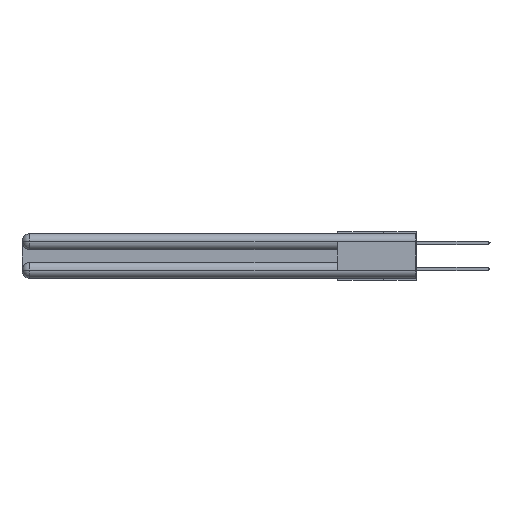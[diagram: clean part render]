
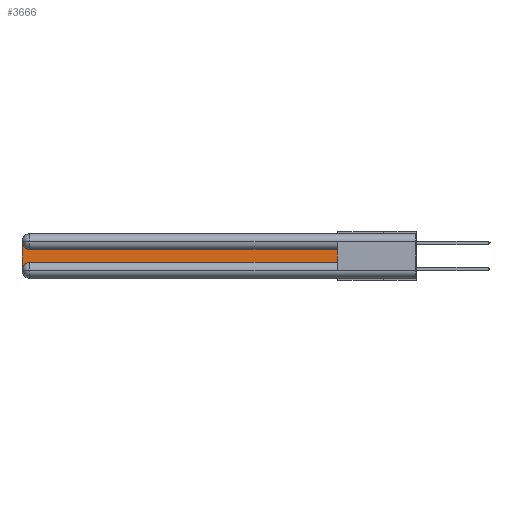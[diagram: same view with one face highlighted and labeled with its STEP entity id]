
A CAD part, left-side view. The second image highlights one B-rep face of the part: STEP entity #3666.
In plain terms, the highlighted planar face has unit normal (-1, 0, 0).
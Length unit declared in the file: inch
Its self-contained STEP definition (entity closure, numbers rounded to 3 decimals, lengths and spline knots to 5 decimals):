
#105 = CARTESIAN_POINT ( 'NONE',  ( 0.075, 2.94, -0.2775 ) ) ;
#425 = CIRCLE ( 'NONE', #22942, 0.06 ) ;
#796 = EDGE_CURVE ( 'NONE', #21981, #18552, #19063, .T. ) ;
#1457 = CARTESIAN_POINT ( 'NONE',  ( 0.075, 0.6, -0.2175 ) ) ;
#1483 = ORIENTED_EDGE ( 'NONE', *, *, #12545, .T. ) ;
#2326 = PLANE ( 'NONE',  #20164 ) ;
#3666 = ADVANCED_FACE ( 'NONE', ( #7728 ), #2326, .F. ) ;
#4022 = LINE ( 'NONE', #29807, #31252 ) ;
#4685 = DIRECTION ( 'NONE',  ( 0., 0., 1. ) ) ;
#5792 = DIRECTION ( 'NONE',  ( 1., 0., 0. ) ) ;
#7728 = FACE_OUTER_BOUND ( 'NONE', #14216, .T. ) ;
#8136 = EDGE_CURVE ( 'NONE', #31898, #27687, #425, .T. ) ;
#9173 = ORIENTED_EDGE ( 'NONE', *, *, #28149, .T. ) ;
#10000 = ORIENTED_EDGE ( 'NONE', *, *, #17375, .T. ) ;
#10413 = DIRECTION ( 'NONE',  ( 0., 0., -1. ) ) ;
#10922 = CARTESIAN_POINT ( 'NONE',  ( 0.075, 2.94, -0.2175 ) ) ;
#12545 = EDGE_CURVE ( 'NONE', #21343, #21981, #31211, .T. ) ;
#14216 = EDGE_LOOP ( 'NONE', ( #10000, #31484, #20580, #1483, #27017, #9173 ) ) ;
#15577 = DIRECTION ( 'NONE',  ( 1., 0., 0. ) ) ;
#16158 = CARTESIAN_POINT ( 'NONE',  ( 0.075, 0.6, -0.1225 ) ) ;
#17375 = EDGE_CURVE ( 'NONE', #26164, #31898, #23611, .T. ) ;
#18552 = VERTEX_POINT ( 'NONE', #1457 ) ;
#18980 = DIRECTION ( 'NONE',  ( 0., -1., 0. ) ) ;
#19063 = LINE ( 'NONE', #24415, #30120 ) ;
#19145 = DIRECTION ( 'NONE',  ( 0., 0., -1. ) ) ;
#19753 = CARTESIAN_POINT ( 'NONE',  ( 0.075, 3., -0.2775 ) ) ;
#19995 = CARTESIAN_POINT ( 'NONE',  ( 0.075, 3., -0.2175 ) ) ;
#20120 = DIRECTION ( 'NONE',  ( 0., 0., -1. ) ) ;
#20164 = AXIS2_PLACEMENT_3D ( 'NONE', #32639, #32169, #10413 ) ;
#20580 = ORIENTED_EDGE ( 'NONE', *, *, #24477, .T. ) ;
#21343 = VERTEX_POINT ( 'NONE', #19753 ) ;
#21544 = CARTESIAN_POINT ( 'NONE',  ( 0.075, 0.6, -0.1225 ) ) ;
#21981 = VERTEX_POINT ( 'NONE', #10922 ) ;
#22942 = AXIS2_PLACEMENT_3D ( 'NONE', #23781, #15577, #34905 ) ;
#23611 = LINE ( 'NONE', #16158, #25318 ) ;
#23781 = CARTESIAN_POINT ( 'NONE',  ( 0.075, 2.94, -0.0625 ) ) ;
#24415 = CARTESIAN_POINT ( 'NONE',  ( 0.075, 0.6, -0.2175 ) ) ;
#24477 = EDGE_CURVE ( 'NONE', #27687, #21343, #34116, .T. ) ;
#25318 = VECTOR ( 'NONE', #34889, 39.37008 ) ;
#25767 = AXIS2_PLACEMENT_3D ( 'NONE', #105, #5792, #19145 ) ;
#26164 = VERTEX_POINT ( 'NONE', #21544 ) ;
#27017 = ORIENTED_EDGE ( 'NONE', *, *, #796, .T. ) ;
#27687 = VERTEX_POINT ( 'NONE', #28642 ) ;
#28149 = EDGE_CURVE ( 'NONE', #18552, #26164, #4022, .T. ) ;
#28642 = CARTESIAN_POINT ( 'NONE',  ( 0.075, 3., -0.0625 ) ) ;
#29055 = CARTESIAN_POINT ( 'NONE',  ( 0.075, 2.94, -0.1225 ) ) ;
#29807 = CARTESIAN_POINT ( 'NONE',  ( 0.075, 0.6, -0.2175 ) ) ;
#30120 = VECTOR ( 'NONE', #18980, 39.37008 ) ;
#30300 = VECTOR ( 'NONE', #20120, 39.37008 ) ;
#31211 = CIRCLE ( 'NONE', #25767, 0.06 ) ;
#31252 = VECTOR ( 'NONE', #4685, 39.37008 ) ;
#31484 = ORIENTED_EDGE ( 'NONE', *, *, #8136, .T. ) ;
#31898 = VERTEX_POINT ( 'NONE', #29055 ) ;
#32169 = DIRECTION ( 'NONE',  ( 1., 0., 0. ) ) ;
#32639 = CARTESIAN_POINT ( 'NONE',  ( 0.075, 3., -0.1225 ) ) ;
#34116 = LINE ( 'NONE', #19995, #30300 ) ;
#34889 = DIRECTION ( 'NONE',  ( 0., 1., 0. ) ) ;
#34905 = DIRECTION ( 'NONE',  ( 0., 0., -1. ) ) ;
